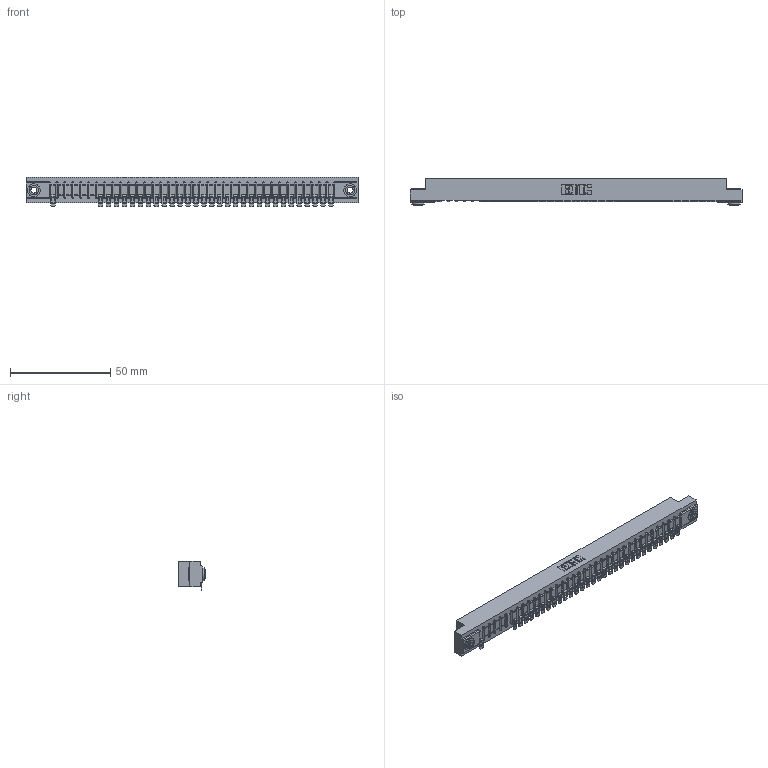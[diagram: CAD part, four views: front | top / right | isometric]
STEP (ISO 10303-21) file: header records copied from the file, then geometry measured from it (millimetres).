
FILE_DESCRIPTION (( 'STEP AP203' ), '1' );
FILE_NAME ('357-036-554-103.STEP', '2018-08-10T05:55:57', ( '' ), ( '' ), 'SwSTEP 2.0', 'SolidWorks 2016', '' );
FILE_SCHEMA (( 'CONFIG_CONTROL_DESIGN' ));
Length unit declared in the file: inch
Products named in the file (4): 357-036-554-103; 307 Part_.156 Dia Mounting Holes; 307-290-002_554; 345-250-002_345-250-002-102
Assembly tree (34 placements, depth 2):
  357-036-554-103
    307 Part_.156 Dia Mounting Holes
    307-290-002_554  x31
    345-250-002_345-250-002-102  x2
Bounding box: 165.66 x 13.36 x 14.52 mm (x, y, z)
Volume: 17550.6 mm3; surface area: 21377.9 mm2
Topology: 34 solids, 34 shells, 2818 faces, 8598 edges, 5628 vertices
Faces by surface type: plane 1580, cylinder 1156, sphere 74, cone 8
Entity records: 33472 total; most frequent: CARTESIAN_POINT 5646, ORIENTED_EDGE 5632, DIRECTION 5504, EDGE_CURVE 2816, VECTOR 2140, LINE 2140, VERTEX_POINT 1824, AXIS2_PLACEMENT_3D 1682
